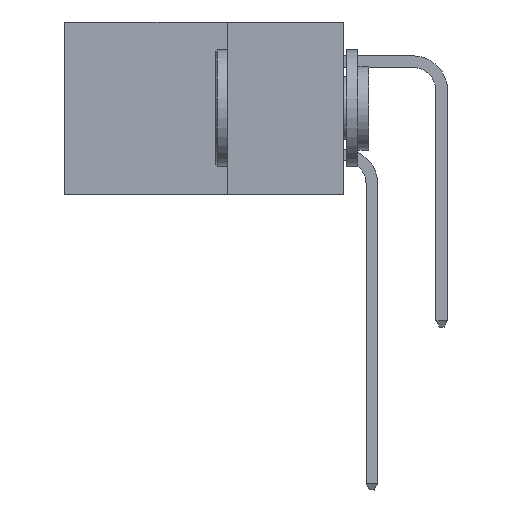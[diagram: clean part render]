
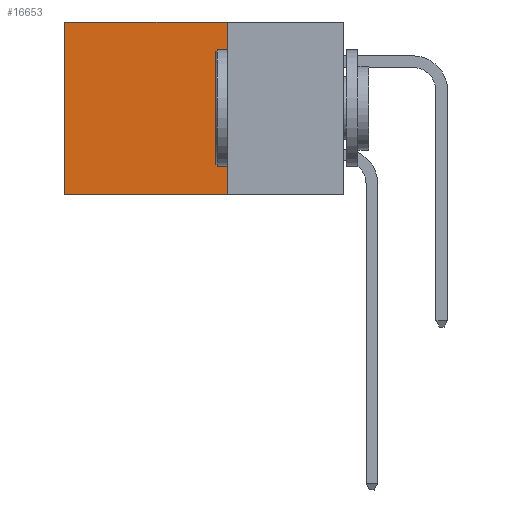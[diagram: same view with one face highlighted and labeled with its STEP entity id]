
A CAD part, left-side view. The second image highlights one B-rep face of the part: STEP entity #16653.
In plain terms, the highlighted planar face has unit normal (-1, 0, 0).
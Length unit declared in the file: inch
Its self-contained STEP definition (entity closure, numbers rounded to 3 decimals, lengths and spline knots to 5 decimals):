
#114 = CARTESIAN_POINT ( 'NONE',  ( 0.298, 0.25, 0. ) ) ;
#1257 = EDGE_CURVE ( 'NONE', #5286, #13193, #26894, .T. ) ;
#1846 = AXIS2_PLACEMENT_3D ( 'NONE', #15990, #15759, #30885 ) ;
#2766 = DIRECTION ( 'NONE',  ( 0., 0., -1. ) ) ;
#4036 = EDGE_CURVE ( 'NONE', #30666, #16925, #32436, .T. ) ;
#4107 = DIRECTION ( 'NONE',  ( 0., 1., 0. ) ) ;
#4390 = VECTOR ( 'NONE', #2766, 39.37008 ) ;
#5286 = VERTEX_POINT ( 'NONE', #18743 ) ;
#5808 = VECTOR ( 'NONE', #13449, 39.37008 ) ;
#6348 = DIRECTION ( 'NONE',  ( 0., 0., -1. ) ) ;
#6727 = VECTOR ( 'NONE', #4107, 39.37008 ) ;
#6787 = CARTESIAN_POINT ( 'NONE',  ( 0.298, 0.25, -0.37 ) ) ;
#10753 = LINE ( 'NONE', #6787, #6727 ) ;
#10939 = CARTESIAN_POINT ( 'NONE',  ( 0.298, 0.6, -0.37 ) ) ;
#11411 = CARTESIAN_POINT ( 'NONE',  ( 0.298, 0.25, -0.37 ) ) ;
#12762 = CARTESIAN_POINT ( 'NONE',  ( 0.298, 0.25, 0. ) ) ;
#12989 = LINE ( 'NONE', #24025, #5808 ) ;
#13050 = EDGE_CURVE ( 'NONE', #30666, #5286, #12989, .T. ) ;
#13193 = VERTEX_POINT ( 'NONE', #10939 ) ;
#13449 = DIRECTION ( 'NONE',  ( 0., 1., 0. ) ) ;
#15759 = DIRECTION ( 'NONE',  ( 1., 0., 0. ) ) ;
#15990 = CARTESIAN_POINT ( 'NONE',  ( 0.298, 0.25, 0. ) ) ;
#16092 = EDGE_LOOP ( 'NONE', ( #18974, #17199, #31046, #31216 ) ) ;
#16276 = EDGE_CURVE ( 'NONE', #16925, #13193, #10753, .T. ) ;
#16653 = ADVANCED_FACE ( 'NONE', ( #22021 ), #31085, .F. ) ;
#16925 = VERTEX_POINT ( 'NONE', #11411 ) ;
#17199 = ORIENTED_EDGE ( 'NONE', *, *, #16276, .F. ) ;
#18743 = CARTESIAN_POINT ( 'NONE',  ( 0.298, 0.6, 0. ) ) ;
#18974 = ORIENTED_EDGE ( 'NONE', *, *, #1257, .T. ) ;
#20138 = VECTOR ( 'NONE', #6348, 39.37008 ) ;
#21618 = CARTESIAN_POINT ( 'NONE',  ( 0.298, 0.6, 0. ) ) ;
#22021 = FACE_OUTER_BOUND ( 'NONE', #16092, .T. ) ;
#24025 = CARTESIAN_POINT ( 'NONE',  ( 0.298, 0.25, 0. ) ) ;
#26894 = LINE ( 'NONE', #21618, #20138 ) ;
#30666 = VERTEX_POINT ( 'NONE', #12762 ) ;
#30885 = DIRECTION ( 'NONE',  ( 0., 0., -1. ) ) ;
#31046 = ORIENTED_EDGE ( 'NONE', *, *, #4036, .F. ) ;
#31085 = PLANE ( 'NONE',  #1846 ) ;
#31216 = ORIENTED_EDGE ( 'NONE', *, *, #13050, .T. ) ;
#32436 = LINE ( 'NONE', #114, #4390 ) ;
